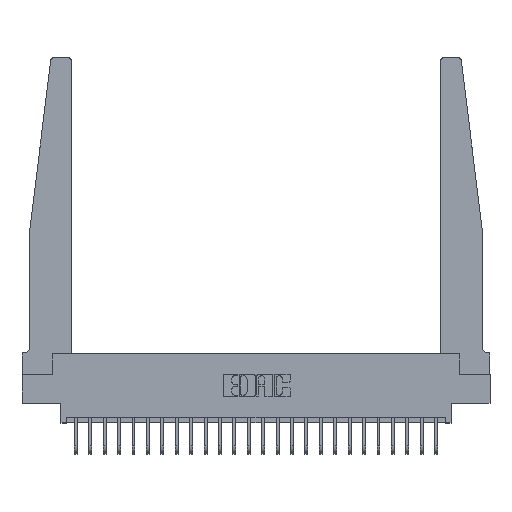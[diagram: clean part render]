
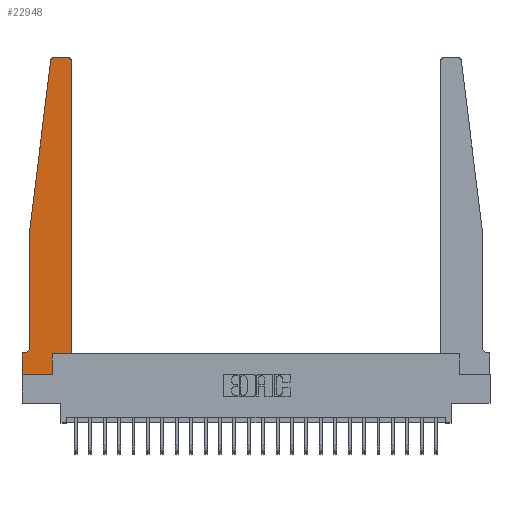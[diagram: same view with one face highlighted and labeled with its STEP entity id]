
A CAD part, top view. The second image highlights one B-rep face of the part: STEP entity #22948.
In plain terms, the highlighted planar face has unit normal (0, 0, 1).
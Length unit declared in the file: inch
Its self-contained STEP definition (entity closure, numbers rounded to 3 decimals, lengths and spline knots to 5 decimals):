
#187 = DIRECTION ( 'NONE',  ( 0., -1., 0. ) ) ;
#1083 = VERTEX_POINT ( 'NONE', #13008 ) ;
#1245 = EDGE_CURVE ( 'NONE', #18051, #23686, #1794, .T. ) ;
#1281 = EDGE_CURVE ( 'NONE', #20518, #10941, #3909, .T. ) ;
#1656 = VERTEX_POINT ( 'NONE', #6261 ) ;
#1794 = LINE ( 'NONE', #22217, #25567 ) ;
#1947 = EDGE_CURVE ( 'NONE', #1656, #14810, #12102, .T. ) ;
#1962 = VECTOR ( 'NONE', #6057, 39.37008 ) ;
#2488 = EDGE_CURVE ( 'NONE', #23686, #13057, #16566, .T. ) ;
#2564 = CARTESIAN_POINT ( 'NONE',  ( 0., 0., 0.37 ) ) ;
#2862 = CIRCLE ( 'NONE', #17741, 0.03 ) ;
#3720 = VERTEX_POINT ( 'NONE', #19769 ) ;
#3909 = LINE ( 'NONE', #20120, #5720 ) ;
#3918 = VECTOR ( 'NONE', #23262, 39.37008 ) ;
#4252 = ORIENTED_EDGE ( 'NONE', *, *, #17268, .T. ) ;
#4268 = VECTOR ( 'NONE', #17193, 39.37008 ) ;
#4292 = DIRECTION ( 'NONE',  ( 0., 1., 0. ) ) ;
#4607 = AXIS2_PLACEMENT_3D ( 'NONE', #8210, #5530, #15805 ) ;
#4702 = DIRECTION ( 'NONE',  ( 1., 0., 0. ) ) ;
#4707 = DIRECTION ( 'NONE',  ( 1., 0., 0. ) ) ;
#5530 = DIRECTION ( 'NONE',  ( 0., 0., 1. ) ) ;
#5720 = VECTOR ( 'NONE', #4292, 39.37008 ) ;
#5979 = EDGE_CURVE ( 'NONE', #1083, #18051, #9076, .T. ) ;
#6013 = VECTOR ( 'NONE', #23291, 39.37008 ) ;
#6057 = DIRECTION ( 'NONE',  ( -1., 0., 0. ) ) ;
#6209 = ORIENTED_EDGE ( 'NONE', *, *, #18664, .T. ) ;
#6261 = CARTESIAN_POINT ( 'NONE',  ( 0., 0.1875, 0.37 ) ) ;
#6324 = CARTESIAN_POINT ( 'NONE',  ( 0.27653, 2.75, 0.37 ) ) ;
#6727 = EDGE_CURVE ( 'NONE', #13057, #1656, #25308, .T. ) ;
#6854 = EDGE_CURVE ( 'NONE', #14810, #21863, #15897, .T. ) ;
#7113 = CARTESIAN_POINT ( 'NONE',  ( 0.065, 0.1875, 0.37 ) ) ;
#7229 = EDGE_CURVE ( 'NONE', #21863, #3720, #15090, .T. ) ;
#7313 = AXIS2_PLACEMENT_3D ( 'NONE', #24054, #23927, #15862 ) ;
#7466 = EDGE_CURVE ( 'NONE', #21834, #1083, #16246, .T. ) ;
#7672 = ORIENTED_EDGE ( 'NONE', *, *, #7466, .T. ) ;
#8210 = CARTESIAN_POINT ( 'NONE',  ( 0., 0.1875, 0.37 ) ) ;
#8376 = ORIENTED_EDGE ( 'NONE', *, *, #2488, .T. ) ;
#8849 = DIRECTION ( 'NONE',  ( 0., 0., 1. ) ) ;
#9076 = LINE ( 'NONE', #21258, #4268 ) ;
#9367 = CARTESIAN_POINT ( 'NONE',  ( 0., 0., 0.37 ) ) ;
#9668 = CARTESIAN_POINT ( 'NONE',  ( 0.25, 2.75, 0.37 ) ) ;
#10326 = LINE ( 'NONE', #20655, #18192 ) ;
#10941 = VERTEX_POINT ( 'NONE', #12078 ) ;
#12078 = CARTESIAN_POINT ( 'NONE',  ( 0.425, 2.72, 0.37 ) ) ;
#12102 = LINE ( 'NONE', #24172, #19662 ) ;
#12328 = DIRECTION ( 'NONE',  ( 0., 0., -1. ) ) ;
#13008 = CARTESIAN_POINT ( 'NONE',  ( 0.24675, 2.72367, 0.37 ) ) ;
#13057 = VERTEX_POINT ( 'NONE', #18556 ) ;
#13861 = CARTESIAN_POINT ( 'NONE',  ( 0.065, 1.25, 0.37 ) ) ;
#14206 = DIRECTION ( 'NONE',  ( -1., 0., 0. ) ) ;
#14271 = EDGE_CURVE ( 'NONE', #15200, #21834, #18174, .T. ) ;
#14456 = CARTESIAN_POINT ( 'NONE',  ( 0.395, 2.72, 0.37 ) ) ;
#14472 = ORIENTED_EDGE ( 'NONE', *, *, #14271, .T. ) ;
#14536 = VECTOR ( 'NONE', #23551, 39.37008 ) ;
#14810 = VERTEX_POINT ( 'NONE', #2564 ) ;
#15090 = LINE ( 'NONE', #23133, #3918 ) ;
#15200 = VERTEX_POINT ( 'NONE', #21239 ) ;
#15805 = DIRECTION ( 'NONE',  ( 1., 0., 0. ) ) ;
#15862 = DIRECTION ( 'NONE',  ( 1., 0., 0. ) ) ;
#15897 = LINE ( 'NONE', #9367, #14536 ) ;
#16246 = CIRCLE ( 'NONE', #7313, 0.03 ) ;
#16456 = CARTESIAN_POINT ( 'NONE',  ( 0.015, 0.2375, 0.37 ) ) ;
#16566 = CIRCLE ( 'NONE', #25442, 0.05 ) ;
#17106 = CARTESIAN_POINT ( 'NONE',  ( 0.425, 0.18, 0.37 ) ) ;
#17193 = DIRECTION ( 'NONE',  ( -0.122, -0.992, 0. ) ) ;
#17268 = EDGE_CURVE ( 'NONE', #10941, #15200, #2862, .T. ) ;
#17462 = CARTESIAN_POINT ( 'NONE',  ( 0.065, 0.2375, 0.37 ) ) ;
#17741 = AXIS2_PLACEMENT_3D ( 'NONE', #14456, #8849, #4702 ) ;
#18051 = VERTEX_POINT ( 'NONE', #13861 ) ;
#18174 = LINE ( 'NONE', #9668, #1962 ) ;
#18192 = VECTOR ( 'NONE', #4707, 39.37008 ) ;
#18556 = CARTESIAN_POINT ( 'NONE',  ( 0.015, 0.1875, 0.37 ) ) ;
#18664 = EDGE_CURVE ( 'NONE', #3720, #20518, #10326, .T. ) ;
#18925 = ORIENTED_EDGE ( 'NONE', *, *, #1245, .T. ) ;
#19130 = ORIENTED_EDGE ( 'NONE', *, *, #1947, .T. ) ;
#19662 = VECTOR ( 'NONE', #22154, 39.37008 ) ;
#19769 = CARTESIAN_POINT ( 'NONE',  ( 0.2605, 0.18, 0.37 ) ) ;
#19864 = ORIENTED_EDGE ( 'NONE', *, *, #5979, .T. ) ;
#19897 = FACE_OUTER_BOUND ( 'NONE', #23627, .T. ) ;
#20120 = CARTESIAN_POINT ( 'NONE',  ( 0.425, 0.18, 0.37 ) ) ;
#20518 = VERTEX_POINT ( 'NONE', #17106 ) ;
#20655 = CARTESIAN_POINT ( 'NONE',  ( 0.425, 0.18, 0.37 ) ) ;
#20691 = ORIENTED_EDGE ( 'NONE', *, *, #6727, .T. ) ;
#21239 = CARTESIAN_POINT ( 'NONE',  ( 0.395, 2.75, 0.37 ) ) ;
#21258 = CARTESIAN_POINT ( 'NONE',  ( 0.065, 1.25, 0.37 ) ) ;
#21834 = VERTEX_POINT ( 'NONE', #6324 ) ;
#21863 = VERTEX_POINT ( 'NONE', #22373 ) ;
#22154 = DIRECTION ( 'NONE',  ( 0., -1., 0. ) ) ;
#22217 = CARTESIAN_POINT ( 'NONE',  ( 0.065, 1.25, 0.37 ) ) ;
#22373 = CARTESIAN_POINT ( 'NONE',  ( 0.2605, 0., 0.37 ) ) ;
#22439 = ORIENTED_EDGE ( 'NONE', *, *, #7229, .T. ) ;
#22948 = ADVANCED_FACE ( 'NONE', ( #19897 ), #24006, .T. ) ;
#23133 = CARTESIAN_POINT ( 'NONE',  ( 0.2605, 0.18, 0.37 ) ) ;
#23262 = DIRECTION ( 'NONE',  ( 0., 1., 0. ) ) ;
#23291 = DIRECTION ( 'NONE',  ( -1., 0., 0. ) ) ;
#23551 = DIRECTION ( 'NONE',  ( 1., 0., 0. ) ) ;
#23627 = EDGE_LOOP ( 'NONE', ( #14472, #7672, #19864, #18925, #8376, #20691, #19130, #23690, #22439, #6209, #25296, #4252 ) ) ;
#23686 = VERTEX_POINT ( 'NONE', #17462 ) ;
#23690 = ORIENTED_EDGE ( 'NONE', *, *, #6854, .T. ) ;
#23927 = DIRECTION ( 'NONE',  ( 0., 0., 1. ) ) ;
#24006 = PLANE ( 'NONE',  #4607 ) ;
#24054 = CARTESIAN_POINT ( 'NONE',  ( 0.27653, 2.72, 0.37 ) ) ;
#24172 = CARTESIAN_POINT ( 'NONE',  ( 0., 0., 0.37 ) ) ;
#25296 = ORIENTED_EDGE ( 'NONE', *, *, #1281, .T. ) ;
#25308 = LINE ( 'NONE', #7113, #6013 ) ;
#25442 = AXIS2_PLACEMENT_3D ( 'NONE', #16456, #12328, #14206 ) ;
#25567 = VECTOR ( 'NONE', #187, 39.37008 ) ;
